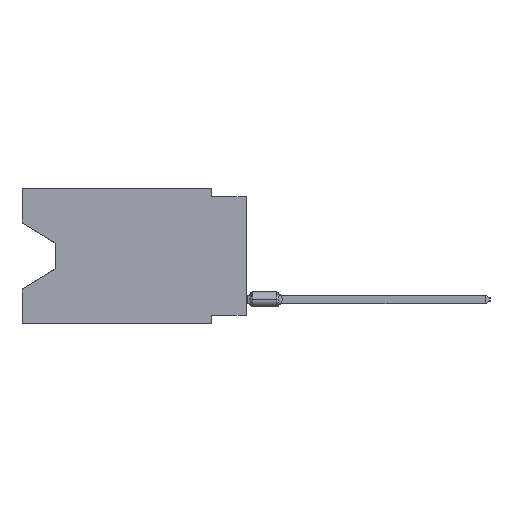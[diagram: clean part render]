
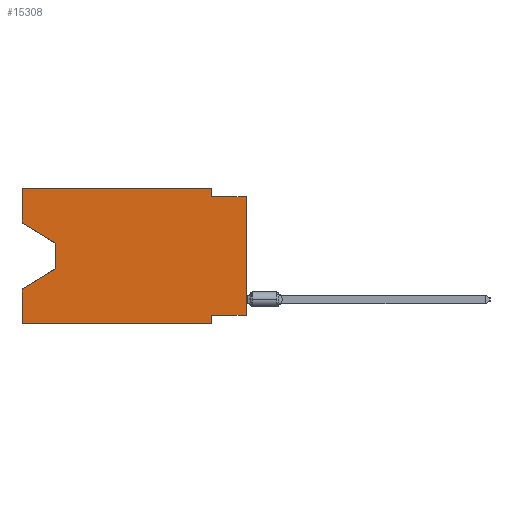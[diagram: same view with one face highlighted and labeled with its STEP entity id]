
A CAD part, left-side view. The second image highlights one B-rep face of the part: STEP entity #15308.
In plain terms, the highlighted planar face has unit normal (-1, 0, 0).
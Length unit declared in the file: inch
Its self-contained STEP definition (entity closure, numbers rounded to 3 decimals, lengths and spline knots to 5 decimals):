
#1618 = VERTEX_POINT ( 'NONE', #56841 ) ;
#4161 = VECTOR ( 'NONE', #47160, 39.37008 ) ;
#4526 = LINE ( 'NONE', #48308, #67069 ) ;
#6136 = DIRECTION ( 'NONE',  ( 0., 0., -1. ) ) ;
#7178 = EDGE_CURVE ( 'NONE', #1618, #73043, #21797, .T. ) ;
#7254 = CARTESIAN_POINT ( 'NONE',  ( 0., 0.1, -0.39 ) ) ;
#12508 = LINE ( 'NONE', #58808, #60812 ) ;
#13209 = EDGE_CURVE ( 'NONE', #46211, #59209, #12508, .T. ) ;
#14332 = VERTEX_POINT ( 'NONE', #41896 ) ;
#15308 = ADVANCED_FACE ( 'NONE', ( #18589 ), #62785, .F. ) ;
#15408 = ORIENTED_EDGE ( 'NONE', *, *, #22470, .T. ) ;
#15520 = VECTOR ( 'NONE', #67249, 39.37008 ) ;
#16053 = CARTESIAN_POINT ( 'NONE',  ( 0., 0.1, -0.365 ) ) ;
#17976 = VECTOR ( 'NONE', #19165, 39.37008 ) ;
#18589 = FACE_OUTER_BOUND ( 'NONE', #82849, .T. ) ;
#18761 = AXIS2_PLACEMENT_3D ( 'NONE', #70401, #56431, #76379 ) ;
#19165 = DIRECTION ( 'NONE',  ( 0., 0., 1. ) ) ;
#20458 = ORIENTED_EDGE ( 'NONE', *, *, #13209, .T. ) ;
#21177 = VECTOR ( 'NONE', #33834, 39.37008 ) ;
#21489 = EDGE_CURVE ( 'NONE', #52719, #83730, #44419, .T. ) ;
#21797 = LINE ( 'NONE', #80847, #15520 ) ;
#22285 = LINE ( 'NONE', #22701, #62433 ) ;
#22470 = EDGE_CURVE ( 'NONE', #73698, #83730, #4526, .T. ) ;
#22701 = CARTESIAN_POINT ( 'NONE',  ( 0., 0.645, -0.10025 ) ) ;
#24058 = DIRECTION ( 'NONE',  ( 0., -1., 0. ) ) ;
#25456 = EDGE_CURVE ( 'NONE', #38556, #73043, #60085, .T. ) ;
#26157 = VERTEX_POINT ( 'NONE', #65741 ) ;
#28709 = LINE ( 'NONE', #41456, #21177 ) ;
#29341 = VERTEX_POINT ( 'NONE', #59863 ) ;
#31508 = LINE ( 'NONE', #32347, #17976 ) ;
#32347 = CARTESIAN_POINT ( 'NONE',  ( 0., 0.645, 0. ) ) ;
#33834 = DIRECTION ( 'NONE',  ( 0., -1., 0. ) ) ;
#34461 = ORIENTED_EDGE ( 'NONE', *, *, #7178, .F. ) ;
#34806 = VERTEX_POINT ( 'NONE', #63646 ) ;
#35041 = CARTESIAN_POINT ( 'NONE',  ( 0., 0., 0. ) ) ;
#35697 = CARTESIAN_POINT ( 'NONE',  ( 0., 0., -0.365 ) ) ;
#38413 = VECTOR ( 'NONE', #63443, 39.37008 ) ;
#38556 = VERTEX_POINT ( 'NONE', #44491 ) ;
#41456 = CARTESIAN_POINT ( 'NONE',  ( 0., 0.645, 0. ) ) ;
#41896 = CARTESIAN_POINT ( 'NONE',  ( 0., 0.645, 0. ) ) ;
#42194 = CARTESIAN_POINT ( 'NONE',  ( 0., 0.1, 0. ) ) ;
#44419 = LINE ( 'NONE', #83088, #56103 ) ;
#44444 = ORIENTED_EDGE ( 'NONE', *, *, #44777, .F. ) ;
#44491 = CARTESIAN_POINT ( 'NONE',  ( 0., 0., -0.365 ) ) ;
#44777 = EDGE_CURVE ( 'NONE', #34806, #1618, #54927, .T. ) ;
#46211 = VERTEX_POINT ( 'NONE', #69349 ) ;
#47160 = DIRECTION ( 'NONE',  ( 0., 1., 0. ) ) ;
#47825 = ORIENTED_EDGE ( 'NONE', *, *, #62917, .T. ) ;
#48308 = CARTESIAN_POINT ( 'NONE',  ( 0., 0.645, -0.39 ) ) ;
#48378 = VECTOR ( 'NONE', #72782, 39.37008 ) ;
#50379 = ORIENTED_EDGE ( 'NONE', *, *, #83855, .F. ) ;
#52719 = VERTEX_POINT ( 'NONE', #16053 ) ;
#54123 = ORIENTED_EDGE ( 'NONE', *, *, #21489, .F. ) ;
#54927 = LINE ( 'NONE', #42194, #48378 ) ;
#56103 = VECTOR ( 'NONE', #77112, 39.37008 ) ;
#56431 = DIRECTION ( 'NONE',  ( 1., 0., 0. ) ) ;
#56841 = CARTESIAN_POINT ( 'NONE',  ( 0., 0.1, -0.025 ) ) ;
#57689 = ORIENTED_EDGE ( 'NONE', *, *, #71259, .F. ) ;
#58808 = CARTESIAN_POINT ( 'NONE',  ( 0., 0.55, -0.158 ) ) ;
#59209 = VERTEX_POINT ( 'NONE', #77721 ) ;
#59863 = CARTESIAN_POINT ( 'NONE',  ( 0., 0.645, -0.28975 ) ) ;
#60085 = LINE ( 'NONE', #35041, #79681 ) ;
#60812 = VECTOR ( 'NONE', #6136, 39.37008 ) ;
#60815 = VECTOR ( 'NONE', #74865, 39.37008 ) ;
#61173 = LINE ( 'NONE', #35697, #4161 ) ;
#62433 = VECTOR ( 'NONE', #80074, 39.37008 ) ;
#62785 = PLANE ( 'NONE',  #18761 ) ;
#62822 = CARTESIAN_POINT ( 'NONE',  ( 0., 0.645, -0.39 ) ) ;
#62917 = EDGE_CURVE ( 'NONE', #26157, #46211, #22285, .T. ) ;
#63443 = DIRECTION ( 'NONE',  ( 0., 0., 1. ) ) ;
#63637 = ORIENTED_EDGE ( 'NONE', *, *, #66055, .F. ) ;
#63646 = CARTESIAN_POINT ( 'NONE',  ( 0., 0.1, 0. ) ) ;
#65741 = CARTESIAN_POINT ( 'NONE',  ( 0., 0.645, -0.10025 ) ) ;
#66055 = EDGE_CURVE ( 'NONE', #26157, #14332, #31508, .T. ) ;
#67069 = VECTOR ( 'NONE', #24058, 39.37008 ) ;
#67249 = DIRECTION ( 'NONE',  ( 0., -1., 0. ) ) ;
#68484 = EDGE_CURVE ( 'NONE', #73698, #29341, #76617, .T. ) ;
#69349 = CARTESIAN_POINT ( 'NONE',  ( 0., 0.55, -0.158 ) ) ;
#70401 = CARTESIAN_POINT ( 'NONE',  ( 0., 0.645, 0. ) ) ;
#71259 = EDGE_CURVE ( 'NONE', #14332, #34806, #28709, .T. ) ;
#71995 = DIRECTION ( 'NONE',  ( 0., 0., 1. ) ) ;
#72402 = ORIENTED_EDGE ( 'NONE', *, *, #68484, .F. ) ;
#72782 = DIRECTION ( 'NONE',  ( 0., 0., -1. ) ) ;
#73043 = VERTEX_POINT ( 'NONE', #73599 ) ;
#73599 = CARTESIAN_POINT ( 'NONE',  ( 0., 0., -0.025 ) ) ;
#73698 = VERTEX_POINT ( 'NONE', #62822 ) ;
#74376 = ORIENTED_EDGE ( 'NONE', *, *, #25456, .T. ) ;
#74433 = ORIENTED_EDGE ( 'NONE', *, *, #79163, .T. ) ;
#74865 = DIRECTION ( 'NONE',  ( 0., 0.855, -0.519 ) ) ;
#75278 = LINE ( 'NONE', #81248, #60815 ) ;
#76379 = DIRECTION ( 'NONE',  ( 0., 0., -1. ) ) ;
#76617 = LINE ( 'NONE', #83009, #38413 ) ;
#77112 = DIRECTION ( 'NONE',  ( 0., 0., -1. ) ) ;
#77721 = CARTESIAN_POINT ( 'NONE',  ( 0., 0.55, -0.232 ) ) ;
#79163 = EDGE_CURVE ( 'NONE', #59209, #29341, #75278, .T. ) ;
#79681 = VECTOR ( 'NONE', #71995, 39.37008 ) ;
#80074 = DIRECTION ( 'NONE',  ( 0., -0.855, -0.519 ) ) ;
#80847 = CARTESIAN_POINT ( 'NONE',  ( 0., 0., -0.025 ) ) ;
#81248 = CARTESIAN_POINT ( 'NONE',  ( 0., 0.55, -0.232 ) ) ;
#82849 = EDGE_LOOP ( 'NONE', ( #47825, #20458, #74433, #72402, #15408, #54123, #50379, #74376, #34461, #44444, #57689, #63637 ) ) ;
#83009 = CARTESIAN_POINT ( 'NONE',  ( 0., 0.645, 0. ) ) ;
#83088 = CARTESIAN_POINT ( 'NONE',  ( 0., 0.1, -0.39 ) ) ;
#83730 = VERTEX_POINT ( 'NONE', #7254 ) ;
#83855 = EDGE_CURVE ( 'NONE', #38556, #52719, #61173, .T. ) ;
